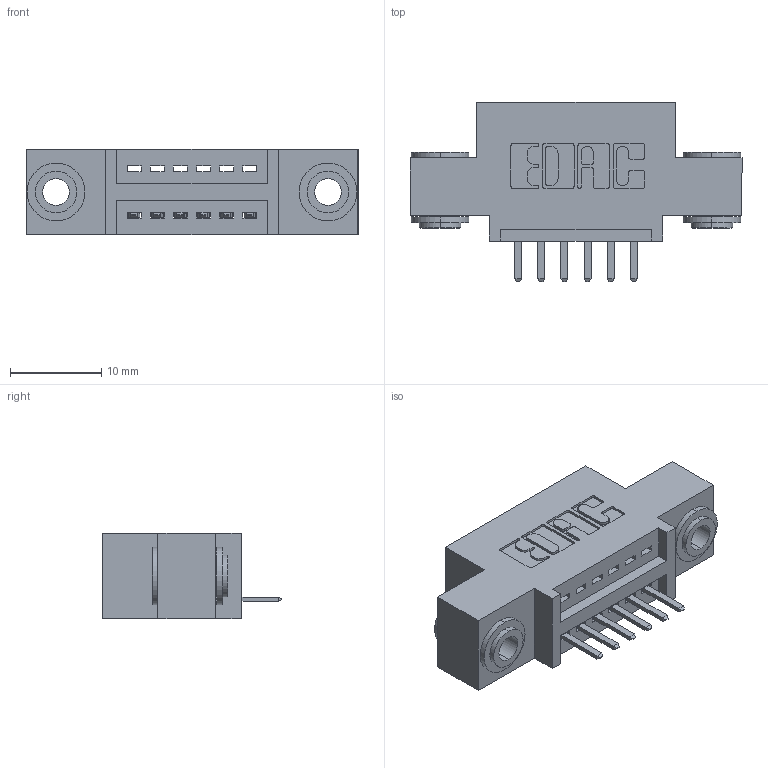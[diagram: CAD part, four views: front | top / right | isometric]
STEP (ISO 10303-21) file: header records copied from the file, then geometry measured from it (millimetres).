
FILE_DESCRIPTION (( 'STEP AP203' ), '1' );
FILE_NAME ('345-006-520-403.STEP', '2018-08-16T23:07:00', ( '' ), ( '' ), 'SwSTEP 2.0', 'SolidWorks 2016', '' );
FILE_SCHEMA (( 'CONFIG_CONTROL_DESIGN' ));
Length unit declared in the file: inch
Products named in the file (4): 345-292-001_345-293-120; 345-250-002_345-250-002-102; 345-006-520-403; 345 Part_0.110 Offset - 0.156 Dia-TH
Assembly tree (9 placements, depth 2):
  345-006-520-403
    345 Part_0.110 Offset - 0.156 Dia-TH
    345-292-001_345-293-120  x6
    345-250-002_345-250-002-102  x2
Bounding box: 36.45 x 19.68 x 9.4 mm (x, y, z)
Volume: 3095.8 mm3; surface area: 3864.7 mm2
Topology: 9 solids, 9 shells, 540 faces, 1533 edges, 1002 vertices
Faces by surface type: plane 346, cylinder 186, cone 8
Entity records: 10258 total; most frequent: CARTESIAN_POINT 1769, ORIENTED_EDGE 1690, DIRECTION 1615, EDGE_CURVE 845, LINE 661, VECTOR 661, VERTEX_POINT 558, AXIS2_PLACEMENT_3D 477
